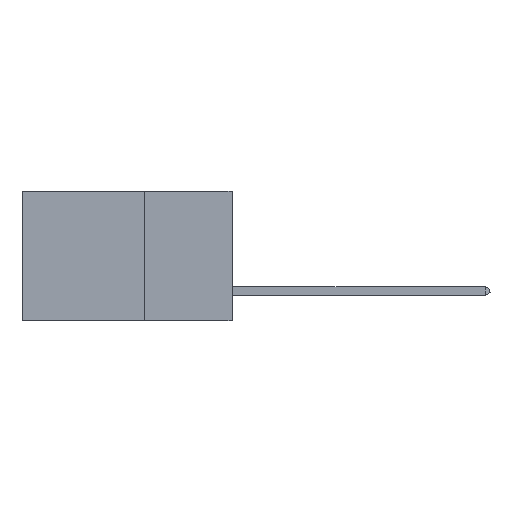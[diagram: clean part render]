
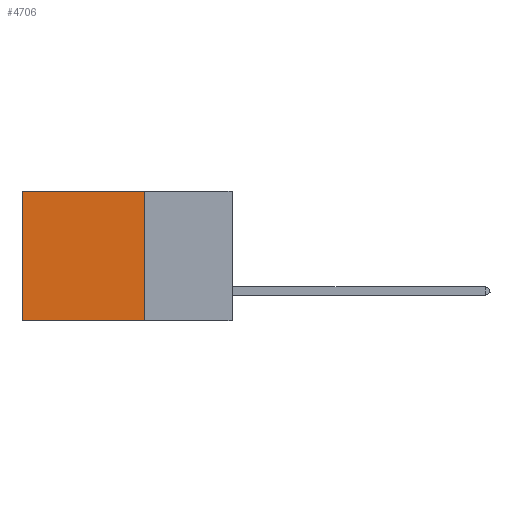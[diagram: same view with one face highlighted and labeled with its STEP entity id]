
A CAD part, left-side view. The second image highlights one B-rep face of the part: STEP entity #4706.
In plain terms, the highlighted planar face has unit normal (-1, 0, 0).
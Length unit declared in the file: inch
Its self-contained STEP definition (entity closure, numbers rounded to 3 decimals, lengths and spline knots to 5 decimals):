
#1336 = DIRECTION ( 'NONE',  ( 1., 0., 0. ) ) ;
#1525 = LINE ( 'NONE', #13951, #20030 ) ;
#4706 = ADVANCED_FACE ( 'NONE', ( #10470 ), #46744, .F. ) ;
#4984 = CARTESIAN_POINT ( 'NONE',  ( 0.2875, 0.25, 0. ) ) ;
#5784 = EDGE_CURVE ( 'NONE', #23549, #18821, #21108, .T. ) ;
#6654 = EDGE_CURVE ( 'NONE', #8454, #16362, #48916, .T. ) ;
#8454 = VERTEX_POINT ( 'NONE', #40289 ) ;
#10037 = ORIENTED_EDGE ( 'NONE', *, *, #34509, .T. ) ;
#10354 = LINE ( 'NONE', #14145, #38920 ) ;
#10470 = FACE_OUTER_BOUND ( 'NONE', #16669, .T. ) ;
#10967 = VECTOR ( 'NONE', #21246, 39.37008 ) ;
#13951 = CARTESIAN_POINT ( 'NONE',  ( 0.2875, 0.25, -0.37 ) ) ;
#14145 = CARTESIAN_POINT ( 'NONE',  ( 0.2875, 0.25, 0. ) ) ;
#14578 = CARTESIAN_POINT ( 'NONE',  ( 0.2875, 0.6, 0. ) ) ;
#14919 = DIRECTION ( 'NONE',  ( 0., 0., -1. ) ) ;
#16345 = DIRECTION ( 'NONE',  ( 0., 0., -1. ) ) ;
#16362 = VERTEX_POINT ( 'NONE', #34877 ) ;
#16669 = EDGE_LOOP ( 'NONE', ( #22424, #29846, #21377, #10037 ) ) ;
#18821 = VERTEX_POINT ( 'NONE', #48778 ) ;
#20030 = VECTOR ( 'NONE', #21774, 39.37008 ) ;
#21108 = LINE ( 'NONE', #32184, #10967 ) ;
#21246 = DIRECTION ( 'NONE',  ( 0., 0., -1. ) ) ;
#21377 = ORIENTED_EDGE ( 'NONE', *, *, #5784, .F. ) ;
#21774 = DIRECTION ( 'NONE',  ( 0., 1., 0. ) ) ;
#22424 = ORIENTED_EDGE ( 'NONE', *, *, #6654, .T. ) ;
#23356 = CARTESIAN_POINT ( 'NONE',  ( 0.2875, 0.25, 0. ) ) ;
#23549 = VERTEX_POINT ( 'NONE', #23356 ) ;
#26604 = EDGE_CURVE ( 'NONE', #18821, #16362, #1525, .T. ) ;
#29846 = ORIENTED_EDGE ( 'NONE', *, *, #26604, .F. ) ;
#32184 = CARTESIAN_POINT ( 'NONE',  ( 0.2875, 0.25, 0. ) ) ;
#34509 = EDGE_CURVE ( 'NONE', #23549, #8454, #10354, .T. ) ;
#34877 = CARTESIAN_POINT ( 'NONE',  ( 0.2875, 0.6, -0.37 ) ) ;
#38920 = VECTOR ( 'NONE', #48542, 39.37008 ) ;
#40289 = CARTESIAN_POINT ( 'NONE',  ( 0.2875, 0.6, 0. ) ) ;
#44120 = VECTOR ( 'NONE', #14919, 39.37008 ) ;
#46744 = PLANE ( 'NONE',  #46842 ) ;
#46842 = AXIS2_PLACEMENT_3D ( 'NONE', #4984, #1336, #16345 ) ;
#48542 = DIRECTION ( 'NONE',  ( 0., 1., 0. ) ) ;
#48778 = CARTESIAN_POINT ( 'NONE',  ( 0.2875, 0.25, -0.37 ) ) ;
#48916 = LINE ( 'NONE', #14578, #44120 ) ;
